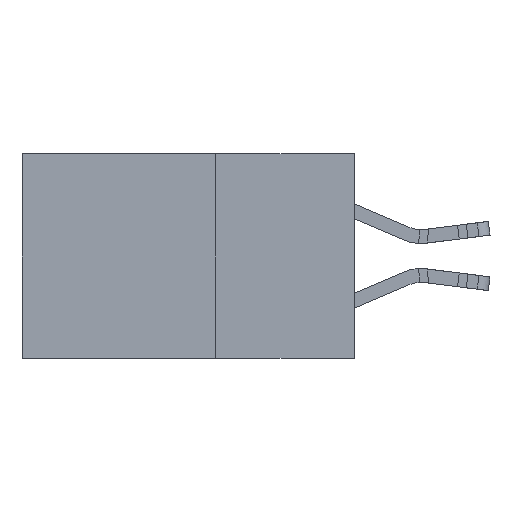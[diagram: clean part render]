
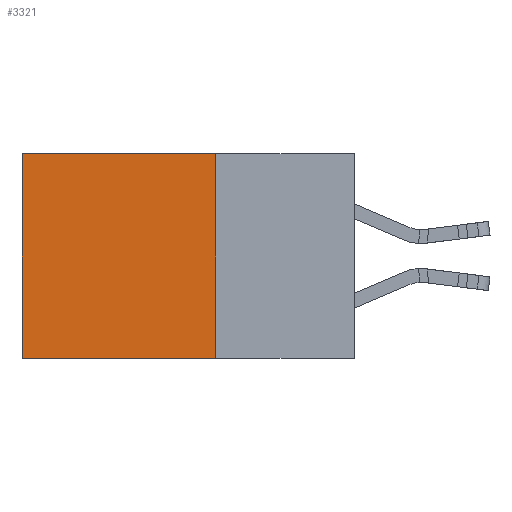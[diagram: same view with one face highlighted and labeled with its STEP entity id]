
A CAD part, left-side view. The second image highlights one B-rep face of the part: STEP entity #3321.
In plain terms, the highlighted planar face has unit normal (-1, 0, 0).
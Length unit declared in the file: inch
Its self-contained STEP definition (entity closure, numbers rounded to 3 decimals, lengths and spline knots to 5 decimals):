
#38 = LINE ( 'NONE', #19275, #5043 ) ;
#274 = ORIENTED_EDGE ( 'NONE', *, *, #7318, .F. ) ;
#402 = CARTESIAN_POINT ( 'NONE',  ( 0.2615, 0.6, -0.37 ) ) ;
#930 = VERTEX_POINT ( 'NONE', #402 ) ;
#983 = DIRECTION ( 'NONE',  ( 0., 1., 0. ) ) ;
#3321 = ADVANCED_FACE ( 'NONE', ( #22329 ), #25290, .F. ) ;
#4054 = VECTOR ( 'NONE', #9647, 39.37008 ) ;
#4563 = ORIENTED_EDGE ( 'NONE', *, *, #8209, .T. ) ;
#5043 = VECTOR ( 'NONE', #11131, 39.37008 ) ;
#6713 = CARTESIAN_POINT ( 'NONE',  ( 0.2615, 0.25, -0.37 ) ) ;
#7318 = EDGE_CURVE ( 'NONE', #25110, #7956, #38, .T. ) ;
#7371 = ORIENTED_EDGE ( 'NONE', *, *, #16473, .T. ) ;
#7956 = VERTEX_POINT ( 'NONE', #6713 ) ;
#8209 = EDGE_CURVE ( 'NONE', #26238, #930, #11253, .T. ) ;
#9647 = DIRECTION ( 'NONE',  ( 0., 0., -1. ) ) ;
#10847 = CARTESIAN_POINT ( 'NONE',  ( 0.2615, 0.6, 0. ) ) ;
#11131 = DIRECTION ( 'NONE',  ( 0., 0., -1. ) ) ;
#11253 = LINE ( 'NONE', #21894, #4054 ) ;
#13544 = CARTESIAN_POINT ( 'NONE',  ( 0.2615, 0.25, 0. ) ) ;
#16228 = EDGE_CURVE ( 'NONE', #7956, #930, #19803, .T. ) ;
#16473 = EDGE_CURVE ( 'NONE', #25110, #26238, #20106, .T. ) ;
#16871 = DIRECTION ( 'NONE',  ( 0., 1., 0. ) ) ;
#18804 = VECTOR ( 'NONE', #983, 39.37008 ) ;
#19145 = VECTOR ( 'NONE', #16871, 39.37008 ) ;
#19275 = CARTESIAN_POINT ( 'NONE',  ( 0.2615, 0.25, -0.37 ) ) ;
#19591 = ORIENTED_EDGE ( 'NONE', *, *, #16228, .F. ) ;
#19803 = LINE ( 'NONE', #21014, #19145 ) ;
#20091 = CARTESIAN_POINT ( 'NONE',  ( 0.2615, 0.25, 0. ) ) ;
#20106 = LINE ( 'NONE', #13544, #18804 ) ;
#21014 = CARTESIAN_POINT ( 'NONE',  ( 0.2615, 0.25, -0.37 ) ) ;
#21894 = CARTESIAN_POINT ( 'NONE',  ( 0.2615, 0.6, -0.37 ) ) ;
#21971 = EDGE_LOOP ( 'NONE', ( #4563, #19591, #274, #7371 ) ) ;
#22329 = FACE_OUTER_BOUND ( 'NONE', #21971, .T. ) ;
#22974 = AXIS2_PLACEMENT_3D ( 'NONE', #24833, #24683, #24648 ) ;
#24648 = DIRECTION ( 'NONE',  ( 0., 0., -1. ) ) ;
#24683 = DIRECTION ( 'NONE',  ( 1., 0., 0. ) ) ;
#24833 = CARTESIAN_POINT ( 'NONE',  ( 0.2615, 0.25, -0.37 ) ) ;
#25110 = VERTEX_POINT ( 'NONE', #20091 ) ;
#25290 = PLANE ( 'NONE',  #22974 ) ;
#26238 = VERTEX_POINT ( 'NONE', #10847 ) ;
